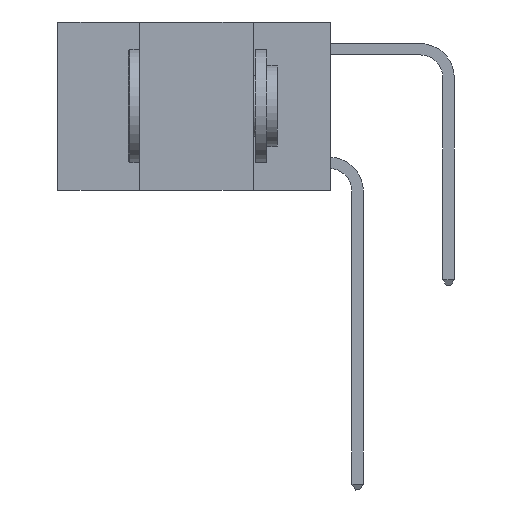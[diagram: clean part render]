
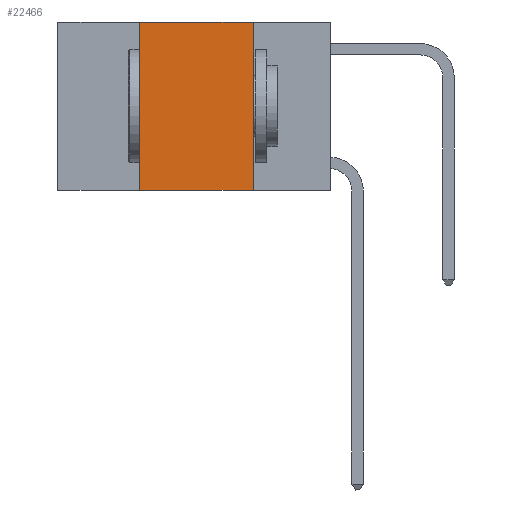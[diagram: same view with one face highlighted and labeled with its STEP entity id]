
A CAD part, left-side view. The second image highlights one B-rep face of the part: STEP entity #22466.
In plain terms, the highlighted planar face has unit normal (-1, 0, 0).
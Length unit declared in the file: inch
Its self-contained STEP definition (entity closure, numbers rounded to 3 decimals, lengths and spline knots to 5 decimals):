
#659 = EDGE_CURVE ( 'NONE', #3095, #4662, #21122, .T. ) ;
#1473 = CARTESIAN_POINT ( 'NONE',  ( 0., 0.42, 0. ) ) ;
#1618 = VERTEX_POINT ( 'NONE', #20483 ) ;
#1964 = VECTOR ( 'NONE', #2111, 39.37008 ) ;
#2111 = DIRECTION ( 'NONE',  ( 0., 0., 1. ) ) ;
#2471 = CARTESIAN_POINT ( 'NONE',  ( 0., 0.42, 0. ) ) ;
#2498 = CARTESIAN_POINT ( 'NONE',  ( 0., 0.17, -0.37 ) ) ;
#3095 = VERTEX_POINT ( 'NONE', #8217 ) ;
#4493 = EDGE_LOOP ( 'NONE', ( #16054, #16364, #19382, #11012 ) ) ;
#4662 = VERTEX_POINT ( 'NONE', #1473 ) ;
#5150 = CARTESIAN_POINT ( 'NONE',  ( 0., 0.6, -0.37 ) ) ;
#5328 = VECTOR ( 'NONE', #14585, 39.37008 ) ;
#6980 = LINE ( 'NONE', #8933, #22871 ) ;
#7745 = FACE_OUTER_BOUND ( 'NONE', #4493, .T. ) ;
#8217 = CARTESIAN_POINT ( 'NONE',  ( 0., 0.42, -0.37 ) ) ;
#8933 = CARTESIAN_POINT ( 'NONE',  ( 0., 0.6, 0. ) ) ;
#9452 = PLANE ( 'NONE',  #17150 ) ;
#11012 = ORIENTED_EDGE ( 'NONE', *, *, #21260, .T. ) ;
#12268 = VERTEX_POINT ( 'NONE', #2498 ) ;
#12998 = LINE ( 'NONE', #5150, #5328 ) ;
#13541 = EDGE_CURVE ( 'NONE', #1618, #12268, #20666, .T. ) ;
#14585 = DIRECTION ( 'NONE',  ( 0., -1., 0. ) ) ;
#15095 = CARTESIAN_POINT ( 'NONE',  ( 0., 0.6, 0. ) ) ;
#15282 = DIRECTION ( 'NONE',  ( 0., 0., -1. ) ) ;
#16054 = ORIENTED_EDGE ( 'NONE', *, *, #13541, .F. ) ;
#16364 = ORIENTED_EDGE ( 'NONE', *, *, #16716, .F. ) ;
#16716 = EDGE_CURVE ( 'NONE', #4662, #1618, #6980, .T. ) ;
#16961 = DIRECTION ( 'NONE',  ( 1., 0., 0. ) ) ;
#17150 = AXIS2_PLACEMENT_3D ( 'NONE', #15095, #16961, #22574 ) ;
#18845 = CARTESIAN_POINT ( 'NONE',  ( 0., 0.17, 0. ) ) ;
#19382 = ORIENTED_EDGE ( 'NONE', *, *, #659, .F. ) ;
#20483 = CARTESIAN_POINT ( 'NONE',  ( 0., 0.17, 0. ) ) ;
#20666 = LINE ( 'NONE', #18845, #23528 ) ;
#21122 = LINE ( 'NONE', #2471, #1964 ) ;
#21260 = EDGE_CURVE ( 'NONE', #3095, #12268, #12998, .T. ) ;
#22048 = DIRECTION ( 'NONE',  ( 0., -1., 0. ) ) ;
#22466 = ADVANCED_FACE ( 'NONE', ( #7745 ), #9452, .F. ) ;
#22574 = DIRECTION ( 'NONE',  ( 0., 0., -1. ) ) ;
#22871 = VECTOR ( 'NONE', #22048, 39.37008 ) ;
#23528 = VECTOR ( 'NONE', #15282, 39.37008 ) ;
